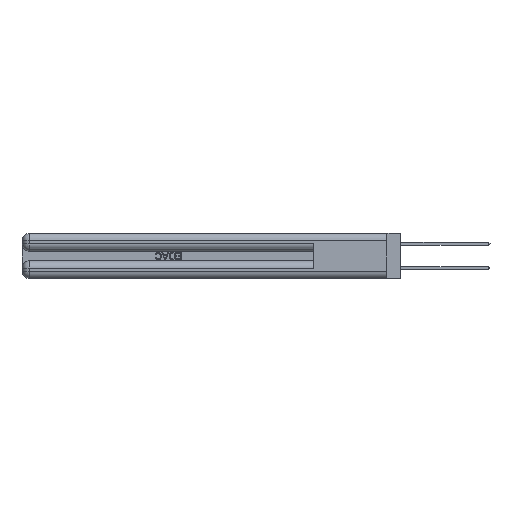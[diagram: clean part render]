
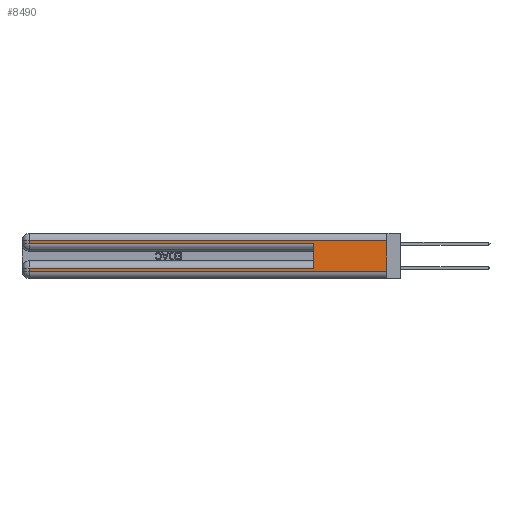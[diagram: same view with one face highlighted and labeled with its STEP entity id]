
A CAD part, left-side view. The second image highlights one B-rep face of the part: STEP entity #8490.
In plain terms, the highlighted planar face has unit normal (-1, 0, 0).
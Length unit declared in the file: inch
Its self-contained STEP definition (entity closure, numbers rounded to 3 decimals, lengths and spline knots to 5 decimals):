
#558 = VERTEX_POINT ( 'NONE', #22185 ) ;
#1549 = DIRECTION ( 'NONE',  ( 0., -1., 0. ) ) ;
#2189 = DIRECTION ( 'NONE',  ( 0., 0., -1. ) ) ;
#2354 = ORIENTED_EDGE ( 'NONE', *, *, #4676, .T. ) ;
#2441 = DIRECTION ( 'NONE',  ( 0., 0., -1. ) ) ;
#4218 = CARTESIAN_POINT ( 'NONE',  ( 0., 0., 0.085 ) ) ;
#4676 = EDGE_CURVE ( 'NONE', #558, #47515, #7185, .T. ) ;
#5625 = LINE ( 'NONE', #10735, #32601 ) ;
#5822 = VERTEX_POINT ( 'NONE', #36560 ) ;
#6028 = CARTESIAN_POINT ( 'NONE',  ( 0., 2.94, 0.37 ) ) ;
#6685 = VECTOR ( 'NONE', #6990, 39.37008 ) ;
#6990 = DIRECTION ( 'NONE',  ( 0., 0., -1. ) ) ;
#7185 = LINE ( 'NONE', #16708, #36523 ) ;
#7261 = FACE_OUTER_BOUND ( 'NONE', #38721, .T. ) ;
#8161 = VECTOR ( 'NONE', #33662, 39.37008 ) ;
#8490 = ADVANCED_FACE ( 'NONE', ( #7261 ), #32107, .F. ) ;
#9658 = ORIENTED_EDGE ( 'NONE', *, *, #22007, .T. ) ;
#9830 = VECTOR ( 'NONE', #15808, 39.37008 ) ;
#10151 = VECTOR ( 'NONE', #16928, 39.37008 ) ;
#10735 = CARTESIAN_POINT ( 'NONE',  ( 0., 0.6, 0.145 ) ) ;
#10924 = CARTESIAN_POINT ( 'NONE',  ( 0., 0., 0.31 ) ) ;
#11937 = CARTESIAN_POINT ( 'NONE',  ( 0., 2.94, 0.085 ) ) ;
#12108 = VERTEX_POINT ( 'NONE', #39388 ) ;
#13586 = CARTESIAN_POINT ( 'NONE',  ( 0., 0., 0.06 ) ) ;
#13598 = EDGE_CURVE ( 'NONE', #21250, #47515, #5625, .T. ) ;
#15542 = ORIENTED_EDGE ( 'NONE', *, *, #35674, .T. ) ;
#15808 = DIRECTION ( 'NONE',  ( 0., 1., 0. ) ) ;
#16481 = EDGE_CURVE ( 'NONE', #12108, #37602, #41591, .T. ) ;
#16708 = CARTESIAN_POINT ( 'NONE',  ( 0., 0., 0.285 ) ) ;
#16928 = DIRECTION ( 'NONE',  ( 0., 1., 0. ) ) ;
#18834 = ORIENTED_EDGE ( 'NONE', *, *, #22851, .T. ) ;
#18970 = VERTEX_POINT ( 'NONE', #11937 ) ;
#19137 = ORIENTED_EDGE ( 'NONE', *, *, #16481, .T. ) ;
#19897 = EDGE_CURVE ( 'NONE', #41458, #5822, #30072, .T. ) ;
#20192 = CARTESIAN_POINT ( 'NONE',  ( 0., 0., 0.31 ) ) ;
#21250 = VERTEX_POINT ( 'NONE', #22545 ) ;
#22007 = EDGE_CURVE ( 'NONE', #21250, #18970, #40915, .T. ) ;
#22185 = CARTESIAN_POINT ( 'NONE',  ( 0., 2.94, 0.285 ) ) ;
#22545 = CARTESIAN_POINT ( 'NONE',  ( 0., 0.6, 0.085 ) ) ;
#22851 = EDGE_CURVE ( 'NONE', #18970, #12108, #36164, .T. ) ;
#26970 = CARTESIAN_POINT ( 'NONE',  ( 0., 0.6, 0.285 ) ) ;
#27851 = CARTESIAN_POINT ( 'NONE',  ( 0., 0., 0.37 ) ) ;
#28529 = LINE ( 'NONE', #6028, #43779 ) ;
#30072 = LINE ( 'NONE', #20192, #10151 ) ;
#30422 = ORIENTED_EDGE ( 'NONE', *, *, #45875, .F. ) ;
#32107 = PLANE ( 'NONE',  #34305 ) ;
#32601 = VECTOR ( 'NONE', #39927, 39.37008 ) ;
#33614 = LINE ( 'NONE', #39940, #6685 ) ;
#33662 = DIRECTION ( 'NONE',  ( 0., -1., 0. ) ) ;
#34305 = AXIS2_PLACEMENT_3D ( 'NONE', #27851, #35721, #43102 ) ;
#35674 = EDGE_CURVE ( 'NONE', #5822, #558, #28529, .T. ) ;
#35721 = DIRECTION ( 'NONE',  ( 1., 0., 0. ) ) ;
#36164 = LINE ( 'NONE', #39548, #44948 ) ;
#36523 = VECTOR ( 'NONE', #1549, 39.37008 ) ;
#36560 = CARTESIAN_POINT ( 'NONE',  ( 0., 2.94, 0.31 ) ) ;
#37602 = VERTEX_POINT ( 'NONE', #13586 ) ;
#37638 = CARTESIAN_POINT ( 'NONE',  ( 0., 0., 0.06 ) ) ;
#38664 = ORIENTED_EDGE ( 'NONE', *, *, #19897, .T. ) ;
#38721 = EDGE_LOOP ( 'NONE', ( #30422, #38664, #15542, #2354, #48403, #9658, #18834, #19137 ) ) ;
#39388 = CARTESIAN_POINT ( 'NONE',  ( 0., 2.94, 0.06 ) ) ;
#39548 = CARTESIAN_POINT ( 'NONE',  ( 0., 2.94, 0.37 ) ) ;
#39927 = DIRECTION ( 'NONE',  ( 0., 0., 1. ) ) ;
#39940 = CARTESIAN_POINT ( 'NONE',  ( 0., 0., 0.37 ) ) ;
#40915 = LINE ( 'NONE', #4218, #9830 ) ;
#41458 = VERTEX_POINT ( 'NONE', #10924 ) ;
#41591 = LINE ( 'NONE', #37638, #8161 ) ;
#43102 = DIRECTION ( 'NONE',  ( 0., 0., -1. ) ) ;
#43779 = VECTOR ( 'NONE', #2441, 39.37008 ) ;
#44948 = VECTOR ( 'NONE', #2189, 39.37008 ) ;
#45875 = EDGE_CURVE ( 'NONE', #41458, #37602, #33614, .T. ) ;
#47515 = VERTEX_POINT ( 'NONE', #26970 ) ;
#48403 = ORIENTED_EDGE ( 'NONE', *, *, #13598, .F. ) ;
